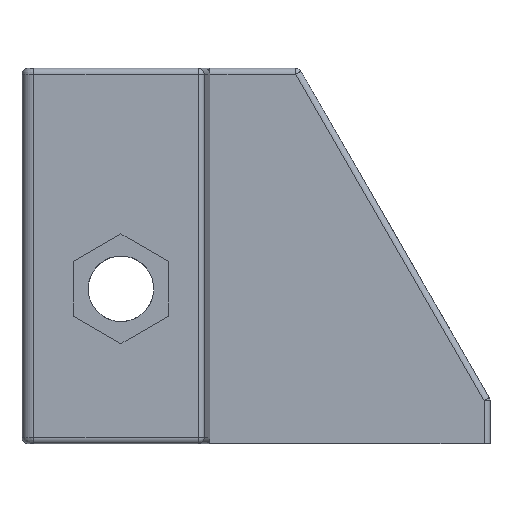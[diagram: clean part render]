
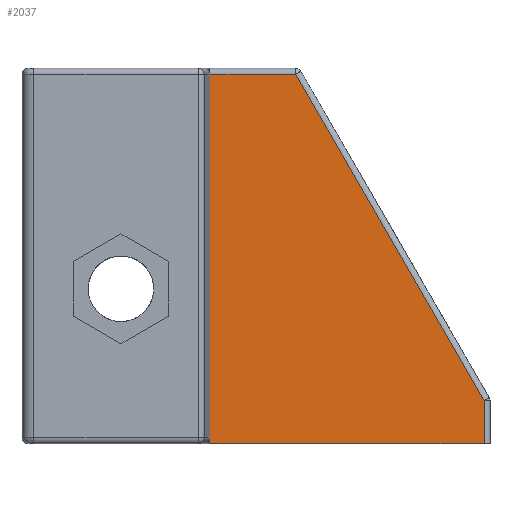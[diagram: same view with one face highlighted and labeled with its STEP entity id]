
A CAD part, left-side view. The second image highlights one B-rep face of the part: STEP entity #2037.
In plain terms, the highlighted planar face has unit normal (-1, 0, 0).
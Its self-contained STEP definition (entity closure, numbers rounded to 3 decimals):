
#375=FACE_OUTER_BOUND('',#509,.T.);
#509=EDGE_LOOP('',(#1768,#1769,#1770,#1771,#1772));
#654=LINE('',#3824,#801);
#661=LINE('',#3847,#808);
#662=LINE('',#3851,#809);
#663=LINE('',#3853,#810);
#664=LINE('',#3854,#811);
#801=VECTOR('',#2901,10.);
#808=VECTOR('',#2928,10.);
#809=VECTOR('',#2933,10.);
#810=VECTOR('',#2934,10.);
#811=VECTOR('',#2935,10.);
#982=VERTEX_POINT('',#3820);
#983=VERTEX_POINT('',#3822);
#989=VERTEX_POINT('',#3846);
#990=VERTEX_POINT('',#3850);
#991=VERTEX_POINT('',#3852);
#1257=EDGE_CURVE('',#983,#982,#654,.T.);
#1268=EDGE_CURVE('',#982,#989,#661,.T.);
#1270=EDGE_CURVE('',#990,#983,#662,.T.);
#1271=EDGE_CURVE('',#991,#990,#663,.T.);
#1272=EDGE_CURVE('',#989,#991,#664,.T.);
#1768=ORIENTED_EDGE('',*,*,#1257,.F.);
#1769=ORIENTED_EDGE('',*,*,#1270,.F.);
#1770=ORIENTED_EDGE('',*,*,#1271,.F.);
#1771=ORIENTED_EDGE('',*,*,#1272,.F.);
#1772=ORIENTED_EDGE('',*,*,#1268,.F.);
#1919=PLANE('',#2305);
#2037=ADVANCED_FACE('',(#375),#1919,.T.);
#2305=AXIS2_PLACEMENT_3D('',#3849,#2931,#2932);
#2901=DIRECTION('',(0.,-1.,0.));
#2928=DIRECTION('',(0.,-0.499,-0.866));
#2931=DIRECTION('center_axis',(-1.,0.,0.));
#2932=DIRECTION('ref_axis',(0.,-1.,0.));
#2933=DIRECTION('',(0.,0.,1.));
#2934=DIRECTION('',(0.,1.,0.));
#2935=DIRECTION('',(0.,0.,-1.));
#3820=CARTESIAN_POINT('',(13.925,-7.711,91.));
#3822=CARTESIAN_POINT('',(13.925,-0.5,91.));
#3824=CARTESIAN_POINT('',(13.925,-2.438,91.));
#3846=CARTESIAN_POINT('',(13.925,-23.5,63.616));
#3847=CARTESIAN_POINT('',(13.925,-21.447,67.178));
#3849=CARTESIAN_POINT('Origin',(13.925,-0.5,60.));
#3850=CARTESIAN_POINT('',(13.925,-0.5,60.));
#3851=CARTESIAN_POINT('',(13.925,-0.5,60.));
#3852=CARTESIAN_POINT('',(13.925,-23.5,60.));
#3853=CARTESIAN_POINT('',(13.925,-24.,60.));
#3854=CARTESIAN_POINT('',(13.925,-23.5,60.));
